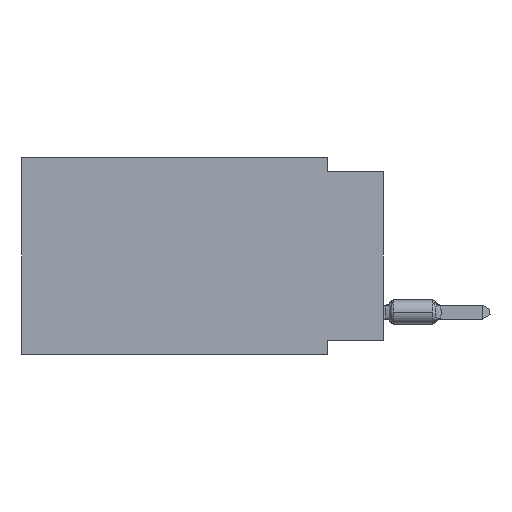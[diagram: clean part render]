
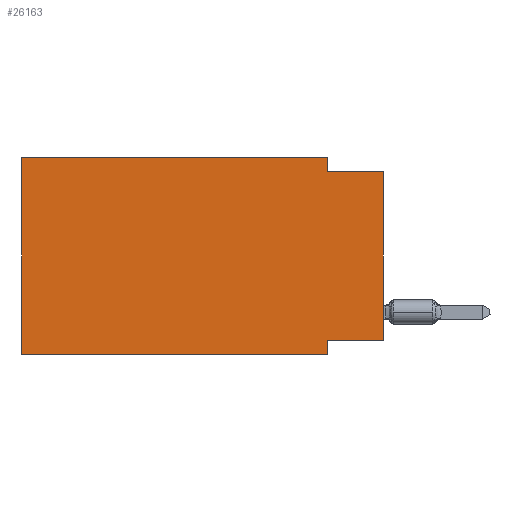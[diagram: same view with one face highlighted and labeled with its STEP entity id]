
A CAD part, left-side view. The second image highlights one B-rep face of the part: STEP entity #26163.
In plain terms, the highlighted planar face has unit normal (-1, 0, 0).
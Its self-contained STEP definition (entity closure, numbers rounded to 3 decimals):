
#1734 = EDGE_CURVE ( 'NONE', #2379, #35734, #12228, .T. ) ;
#2171 = CARTESIAN_POINT ( 'NONE',  ( 0., 0., -0.635 ) ) ;
#2379 = VERTEX_POINT ( 'NONE', #32512 ) ;
#2693 = LINE ( 'NONE', #68620, #59683 ) ;
#2840 = CARTESIAN_POINT ( 'NONE',  ( 0., 16.383, 0. ) ) ;
#6228 = VECTOR ( 'NONE', #7444, 1000. ) ;
#6852 = DIRECTION ( 'NONE',  ( 0., 0., 1. ) ) ;
#7132 = VERTEX_POINT ( 'NONE', #36676 ) ;
#7444 = DIRECTION ( 'NONE',  ( 0., -1., 0. ) ) ;
#8753 = ORIENTED_EDGE ( 'NONE', *, *, #26248, .F. ) ;
#11474 = CARTESIAN_POINT ( 'NONE',  ( 0., 2.54, -8.255 ) ) ;
#12228 = LINE ( 'NONE', #24383, #55784 ) ;
#13299 = CARTESIAN_POINT ( 'NONE',  ( 0., 16.383, 0. ) ) ;
#13430 = EDGE_LOOP ( 'NONE', ( #34678, #21888, #64574, #68726, #56988, #44701, #39791, #8753 ) ) ;
#13653 = CARTESIAN_POINT ( 'NONE',  ( 0., 0., -8.255 ) ) ;
#14848 = AXIS2_PLACEMENT_3D ( 'NONE', #13299, #52007, #18673 ) ;
#17471 = EDGE_CURVE ( 'NONE', #49871, #21350, #26373, .T. ) ;
#18556 = LINE ( 'NONE', #44736, #6228 ) ;
#18673 = DIRECTION ( 'NONE',  ( 0., 0., -1. ) ) ;
#19939 = EDGE_CURVE ( 'NONE', #22782, #68253, #58749, .T. ) ;
#21350 = VERTEX_POINT ( 'NONE', #66237 ) ;
#21575 = CARTESIAN_POINT ( 'NONE',  ( 0., 16.383, 0. ) ) ;
#21888 = ORIENTED_EDGE ( 'NONE', *, *, #51487, .F. ) ;
#22782 = VERTEX_POINT ( 'NONE', #25730 ) ;
#24027 = VECTOR ( 'NONE', #69192, 1000. ) ;
#24032 = FACE_OUTER_BOUND ( 'NONE', #13430, .T. ) ;
#24383 = CARTESIAN_POINT ( 'NONE',  ( 0., 0., 0. ) ) ;
#24798 = CARTESIAN_POINT ( 'NONE',  ( 0., 16.383, -8.89 ) ) ;
#25047 = DIRECTION ( 'NONE',  ( 0., 0., 1. ) ) ;
#25730 = CARTESIAN_POINT ( 'NONE',  ( 0., 16.383, -8.89 ) ) ;
#26163 = ADVANCED_FACE ( 'NONE', ( #24032 ), #57390, .F. ) ;
#26248 = EDGE_CURVE ( 'NONE', #2379, #49871, #52723, .T. ) ;
#26373 = LINE ( 'NONE', #48267, #50262 ) ;
#26737 = DIRECTION ( 'NONE',  ( 0., 0., -1. ) ) ;
#31141 = VECTOR ( 'NONE', #68169, 1000. ) ;
#32512 = CARTESIAN_POINT ( 'NONE',  ( 0., 0., -8.255 ) ) ;
#34678 = ORIENTED_EDGE ( 'NONE', *, *, #1734, .T. ) ;
#35734 = VERTEX_POINT ( 'NONE', #2171 ) ;
#36200 = VECTOR ( 'NONE', #58869, 1000. ) ;
#36676 = CARTESIAN_POINT ( 'NONE',  ( 0., 2.54, -0.635 ) ) ;
#39791 = ORIENTED_EDGE ( 'NONE', *, *, #17471, .F. ) ;
#42023 = CARTESIAN_POINT ( 'NONE',  ( 0., 2.54, 0. ) ) ;
#42515 = EDGE_CURVE ( 'NONE', #44385, #7132, #53489, .T. ) ;
#44385 = VERTEX_POINT ( 'NONE', #62659 ) ;
#44701 = ORIENTED_EDGE ( 'NONE', *, *, #49161, .T. ) ;
#44736 = CARTESIAN_POINT ( 'NONE',  ( 0., 0., -0.635 ) ) ;
#48267 = CARTESIAN_POINT ( 'NONE',  ( 0., 2.54, -8.89 ) ) ;
#49161 = EDGE_CURVE ( 'NONE', #22782, #21350, #56730, .T. ) ;
#49871 = VERTEX_POINT ( 'NONE', #11474 ) ;
#50262 = VECTOR ( 'NONE', #26737, 1000. ) ;
#51487 = EDGE_CURVE ( 'NONE', #7132, #35734, #18556, .T. ) ;
#52007 = DIRECTION ( 'NONE',  ( 1., 0., 0. ) ) ;
#52723 = LINE ( 'NONE', #13653, #24027 ) ;
#53489 = LINE ( 'NONE', #42023, #36200 ) ;
#55784 = VECTOR ( 'NONE', #6852, 1000. ) ;
#56730 = LINE ( 'NONE', #24798, #31141 ) ;
#56988 = ORIENTED_EDGE ( 'NONE', *, *, #19939, .F. ) ;
#57390 = PLANE ( 'NONE',  #14848 ) ;
#57893 = DIRECTION ( 'NONE',  ( 0., -1., 0. ) ) ;
#58459 = VECTOR ( 'NONE', #25047, 1000. ) ;
#58749 = LINE ( 'NONE', #2840, #58459 ) ;
#58869 = DIRECTION ( 'NONE',  ( 0., 0., -1. ) ) ;
#59683 = VECTOR ( 'NONE', #57893, 1000. ) ;
#62659 = CARTESIAN_POINT ( 'NONE',  ( 0., 2.54, 0. ) ) ;
#64574 = ORIENTED_EDGE ( 'NONE', *, *, #42515, .F. ) ;
#66237 = CARTESIAN_POINT ( 'NONE',  ( 0., 2.54, -8.89 ) ) ;
#66386 = EDGE_CURVE ( 'NONE', #68253, #44385, #2693, .T. ) ;
#68169 = DIRECTION ( 'NONE',  ( 0., -1., 0. ) ) ;
#68253 = VERTEX_POINT ( 'NONE', #21575 ) ;
#68620 = CARTESIAN_POINT ( 'NONE',  ( 0., 16.383, 0. ) ) ;
#68726 = ORIENTED_EDGE ( 'NONE', *, *, #66386, .F. ) ;
#69192 = DIRECTION ( 'NONE',  ( 0., 1., 0. ) ) ;
